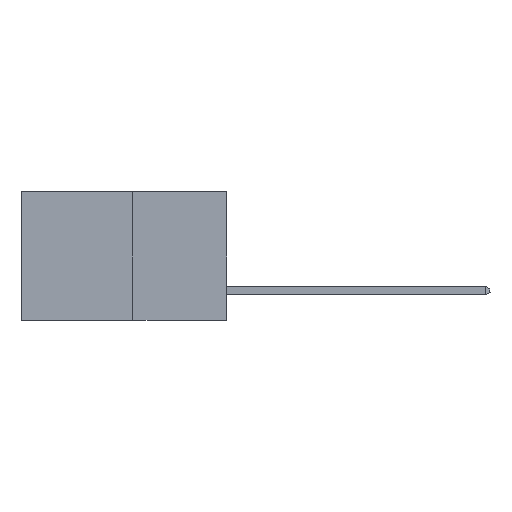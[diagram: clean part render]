
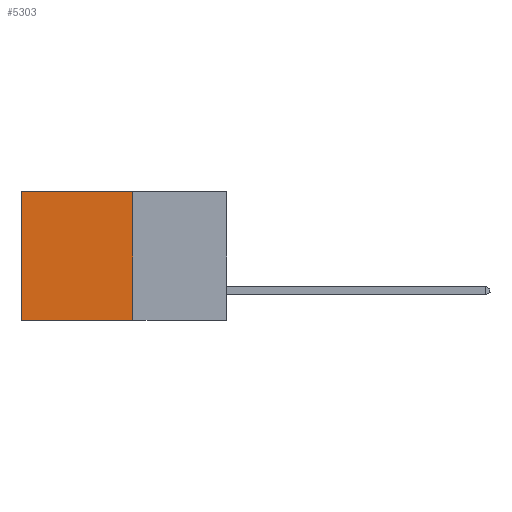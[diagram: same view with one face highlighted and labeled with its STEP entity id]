
A CAD part, left-side view. The second image highlights one B-rep face of the part: STEP entity #5303.
In plain terms, the highlighted planar face has unit normal (-1, 0, 0).
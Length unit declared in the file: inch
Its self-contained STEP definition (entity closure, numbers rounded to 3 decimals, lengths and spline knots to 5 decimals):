
#916 = PLANE ( 'NONE',  #10696 ) ;
#1529 = VERTEX_POINT ( 'NONE', #13797 ) ;
#1780 = LINE ( 'NONE', #4388, #12533 ) ;
#2134 = DIRECTION ( 'NONE',  ( 1., 0., 0. ) ) ;
#2657 = LINE ( 'NONE', #14472, #17049 ) ;
#2999 = CARTESIAN_POINT ( 'NONE',  ( 0.277, 0.27, 0. ) ) ;
#3653 = ORIENTED_EDGE ( 'NONE', *, *, #6155, .T. ) ;
#3942 = VECTOR ( 'NONE', #9603, 39.37008 ) ;
#3973 = EDGE_CURVE ( 'NONE', #14910, #1529, #10856, .T. ) ;
#4375 = LINE ( 'NONE', #16507, #3942 ) ;
#4388 = CARTESIAN_POINT ( 'NONE',  ( 0.277, 0.27, -0.37 ) ) ;
#4510 = DIRECTION ( 'NONE',  ( 0., 1., 0. ) ) ;
#5303 = ADVANCED_FACE ( 'NONE', ( #17506 ), #916, .F. ) ;
#6155 = EDGE_CURVE ( 'NONE', #1529, #6545, #2657, .T. ) ;
#6545 = VERTEX_POINT ( 'NONE', #8999 ) ;
#6688 = ORIENTED_EDGE ( 'NONE', *, *, #14183, .F. ) ;
#8437 = EDGE_CURVE ( 'NONE', #10192, #6545, #1780, .T. ) ;
#8999 = CARTESIAN_POINT ( 'NONE',  ( 0.277, 0.59, -0.37 ) ) ;
#9603 = DIRECTION ( 'NONE',  ( 0., 0., -1. ) ) ;
#10192 = VERTEX_POINT ( 'NONE', #12953 ) ;
#10696 = AXIS2_PLACEMENT_3D ( 'NONE', #17870, #2134, #12183 ) ;
#10856 = LINE ( 'NONE', #15516, #11741 ) ;
#10888 = ORIENTED_EDGE ( 'NONE', *, *, #8437, .F. ) ;
#11741 = VECTOR ( 'NONE', #15466, 39.37008 ) ;
#12183 = DIRECTION ( 'NONE',  ( 0., 0., -1. ) ) ;
#12533 = VECTOR ( 'NONE', #4510, 39.37008 ) ;
#12870 = EDGE_LOOP ( 'NONE', ( #3653, #10888, #6688, #13920 ) ) ;
#12953 = CARTESIAN_POINT ( 'NONE',  ( 0.277, 0.27, -0.37 ) ) ;
#13797 = CARTESIAN_POINT ( 'NONE',  ( 0.277, 0.59, 0. ) ) ;
#13920 = ORIENTED_EDGE ( 'NONE', *, *, #3973, .T. ) ;
#14183 = EDGE_CURVE ( 'NONE', #14910, #10192, #4375, .T. ) ;
#14223 = DIRECTION ( 'NONE',  ( 0., 0., -1. ) ) ;
#14472 = CARTESIAN_POINT ( 'NONE',  ( 0.277, 0.59, -0.37 ) ) ;
#14910 = VERTEX_POINT ( 'NONE', #2999 ) ;
#15466 = DIRECTION ( 'NONE',  ( 0., 1., 0. ) ) ;
#15516 = CARTESIAN_POINT ( 'NONE',  ( 0.277, 0.27, 0. ) ) ;
#16507 = CARTESIAN_POINT ( 'NONE',  ( 0.277, 0.27, -0.37 ) ) ;
#17049 = VECTOR ( 'NONE', #14223, 39.37008 ) ;
#17506 = FACE_OUTER_BOUND ( 'NONE', #12870, .T. ) ;
#17870 = CARTESIAN_POINT ( 'NONE',  ( 0.277, 0.27, -0.37 ) ) ;
